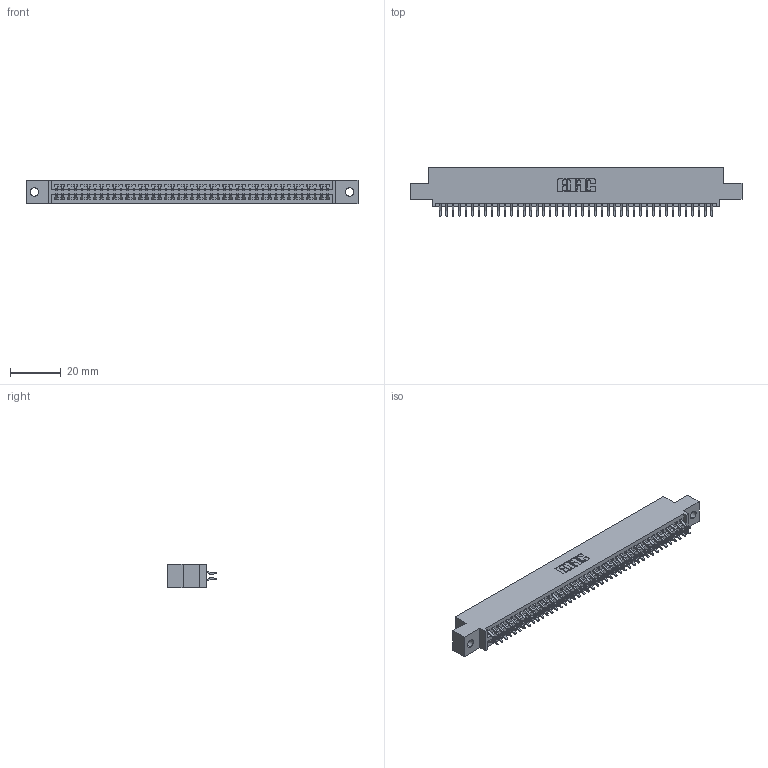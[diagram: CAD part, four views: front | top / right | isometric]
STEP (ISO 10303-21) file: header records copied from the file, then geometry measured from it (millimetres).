
FILE_DESCRIPTION (( 'STEP AP203' ), '1' );
FILE_NAME ('395-086-556-502.STEP', '2018-11-28T22:00:21', ( '' ), ( '' ), 'SwSTEP 2.0', 'SolidWorks 2016', '' );
FILE_SCHEMA (( 'CONFIG_CONTROL_DESIGN' ));
Length unit declared in the file: inch
Products named in the file (3): 345-292-001_556 Tail; 345 Part_0.110 Offset - 0.128 Dia; 395-086-556-502
Assembly tree (87 placements, depth 2):
  395-086-556-502
    345 Part_0.110 Offset - 0.128 Dia
    345-292-001_556 Tail  x86
Bounding box: 130.43 x 19.24 x 9.4 mm (x, y, z)
Volume: 12565.8 mm3; surface area: 18338.6 mm2
Topology: 87 solids, 87 shells, 4946 faces, 14715 edges, 9694 vertices
Faces by surface type: plane 3266, cylinder 1680
Entity records: 33959 total; most frequent: CARTESIAN_POINT 5708, ORIENTED_EDGE 5630, DIRECTION 5019, EDGE_CURVE 2815, VECTOR 2503, LINE 2503, VERTEX_POINT 1874, AXIS2_PLACEMENT_3D 1258
